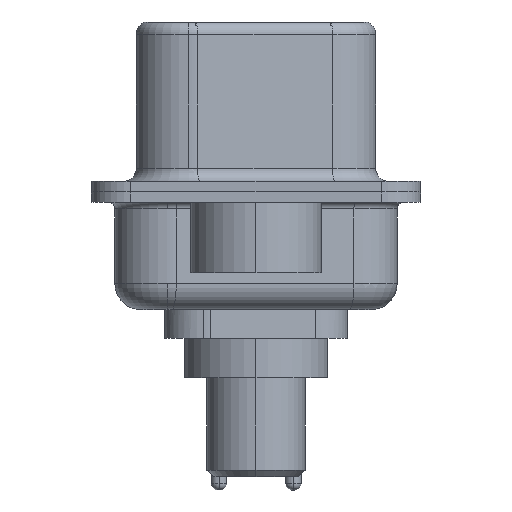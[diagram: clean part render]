
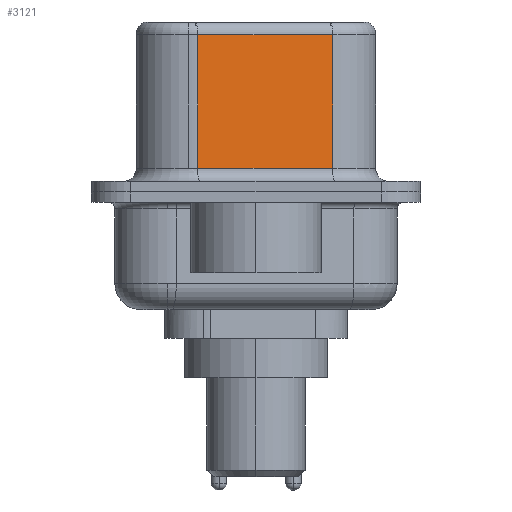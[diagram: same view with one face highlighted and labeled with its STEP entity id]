
A CAD part, left-side view. The second image highlights one B-rep face of the part: STEP entity #3121.
In plain terms, the highlighted planar face has unit normal (-0.985, -0.174, 0).
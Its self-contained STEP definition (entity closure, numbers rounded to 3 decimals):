
#230 = VERTEX_POINT ( 'NONE', #15614 ) ;
#2552 = ORIENTED_EDGE ( 'NONE', *, *, #5553, .F. ) ;
#3121 = ADVANCED_FACE ( 'NONE', ( #4199 ), #4851, .F. ) ;
#3948 = AXIS2_PLACEMENT_3D ( 'NONE', #9890, #9009, #17869 ) ;
#4055 = VECTOR ( 'NONE', #14335, 1000. ) ;
#4199 = FACE_OUTER_BOUND ( 'NONE', #11830, .T. ) ;
#4851 = PLANE ( 'NONE',  #3948 ) ;
#5167 = CARTESIAN_POINT ( 'NONE',  ( 3.67, 2.233, 0.9 ) ) ;
#5552 = LINE ( 'NONE', #16293, #18929 ) ;
#5553 = EDGE_CURVE ( 'NONE', #8822, #230, #18508, .T. ) ;
#5744 = CARTESIAN_POINT ( 'NONE',  ( 4.58, -2.927, 0.9 ) ) ;
#7081 = EDGE_CURVE ( 'NONE', #15750, #14417, #15945, .T. ) ;
#7825 = VECTOR ( 'NONE', #17935, 1000. ) ;
#8364 = LINE ( 'NONE', #5744, #7825 ) ;
#8822 = VERTEX_POINT ( 'NONE', #13059 ) ;
#9009 = DIRECTION ( 'NONE',  ( 0.985, 0.174, 0. ) ) ;
#9890 = CARTESIAN_POINT ( 'NONE',  ( 4.58, -2.927, 6.52 ) ) ;
#10889 = DIRECTION ( 'NONE',  ( -0.174, 0.985, 0. ) ) ;
#11319 = VECTOR ( 'NONE', #12907, 1000. ) ;
#11830 = EDGE_LOOP ( 'NONE', ( #2552, #20204, #19612, #14648 ) ) ;
#11886 = EDGE_CURVE ( 'NONE', #8822, #15750, #5552, .T. ) ;
#12907 = DIRECTION ( 'NONE',  ( 0., 0., -1. ) ) ;
#13059 = CARTESIAN_POINT ( 'NONE',  ( 4.58, -2.927, 6.02 ) ) ;
#13413 = CARTESIAN_POINT ( 'NONE',  ( 3.67, 2.233, 6.52 ) ) ;
#14176 = CARTESIAN_POINT ( 'NONE',  ( 4.58, -2.927, 6.52 ) ) ;
#14335 = DIRECTION ( 'NONE',  ( 0., 0., -1. ) ) ;
#14417 = VERTEX_POINT ( 'NONE', #5167 ) ;
#14648 = ORIENTED_EDGE ( 'NONE', *, *, #20348, .T. ) ;
#15614 = CARTESIAN_POINT ( 'NONE',  ( 4.58, -2.927, 0.9 ) ) ;
#15750 = VERTEX_POINT ( 'NONE', #15814 ) ;
#15814 = CARTESIAN_POINT ( 'NONE',  ( 3.67, 2.233, 6.02 ) ) ;
#15945 = LINE ( 'NONE', #13413, #11319 ) ;
#16293 = CARTESIAN_POINT ( 'NONE',  ( 4.58, -2.927, 6.02 ) ) ;
#17869 = DIRECTION ( 'NONE',  ( -0.174, 0.985, 0. ) ) ;
#17935 = DIRECTION ( 'NONE',  ( 0.174, -0.985, 0. ) ) ;
#18508 = LINE ( 'NONE', #14176, #4055 ) ;
#18929 = VECTOR ( 'NONE', #10889, 1000. ) ;
#19612 = ORIENTED_EDGE ( 'NONE', *, *, #7081, .T. ) ;
#20204 = ORIENTED_EDGE ( 'NONE', *, *, #11886, .T. ) ;
#20348 = EDGE_CURVE ( 'NONE', #14417, #230, #8364, .T. ) ;
